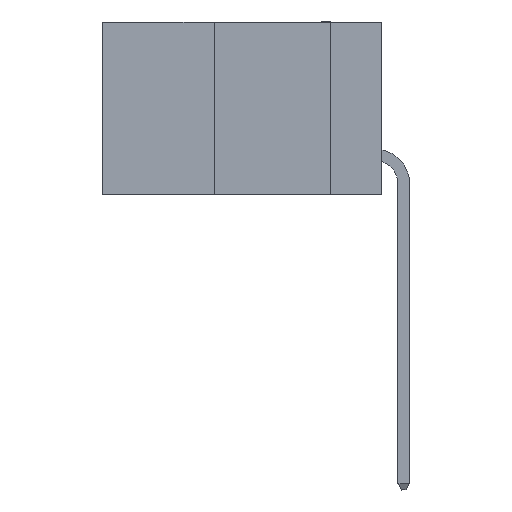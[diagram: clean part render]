
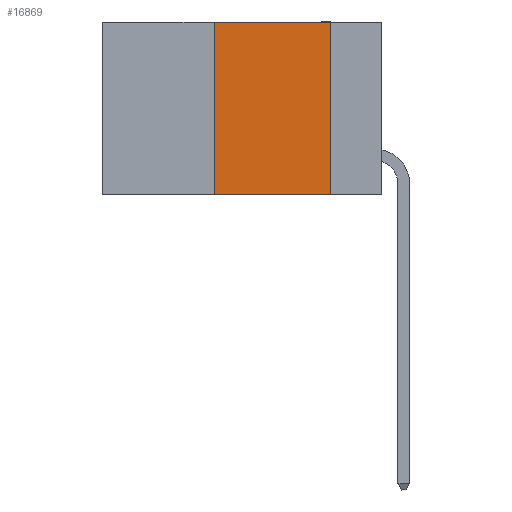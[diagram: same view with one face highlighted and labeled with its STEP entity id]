
A CAD part, left-side view. The second image highlights one B-rep face of the part: STEP entity #16869.
In plain terms, the highlighted planar face has unit normal (-1, 0, 0).
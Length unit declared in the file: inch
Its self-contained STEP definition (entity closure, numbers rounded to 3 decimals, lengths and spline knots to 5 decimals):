
#229 = CARTESIAN_POINT ( 'NONE',  ( 0., 0.36, -0.37 ) ) ;
#3249 = EDGE_CURVE ( 'NONE', #15118, #6403, #12696, .T. ) ;
#6213 = PLANE ( 'NONE',  #23987 ) ;
#6403 = VERTEX_POINT ( 'NONE', #13923 ) ;
#6944 = DIRECTION ( 'NONE',  ( 0., -1., 0. ) ) ;
#7377 = EDGE_LOOP ( 'NONE', ( #34557, #25015, #31800, #25762 ) ) ;
#7876 = CARTESIAN_POINT ( 'NONE',  ( 0., 0.11, 0. ) ) ;
#7880 = VECTOR ( 'NONE', #6944, 39.37008 ) ;
#8492 = EDGE_CURVE ( 'NONE', #6403, #29440, #18945, .T. ) ;
#8942 = DIRECTION ( 'NONE',  ( 0., 0., -1. ) ) ;
#9157 = VECTOR ( 'NONE', #33090, 39.37008 ) ;
#9980 = VERTEX_POINT ( 'NONE', #229 ) ;
#10859 = EDGE_CURVE ( 'NONE', #9980, #15118, #15695, .T. ) ;
#12696 = LINE ( 'NONE', #19470, #9157 ) ;
#13923 = CARTESIAN_POINT ( 'NONE',  ( 0., 0.11, 0. ) ) ;
#15118 = VERTEX_POINT ( 'NONE', #27117 ) ;
#15695 = LINE ( 'NONE', #26704, #30376 ) ;
#16257 = CARTESIAN_POINT ( 'NONE',  ( 0., 0.6, -0.37 ) ) ;
#16719 = VECTOR ( 'NONE', #21004, 39.37008 ) ;
#16869 = ADVANCED_FACE ( 'NONE', ( #17490 ), #6213, .F. ) ;
#17490 = FACE_OUTER_BOUND ( 'NONE', #7377, .T. ) ;
#18259 = DIRECTION ( 'NONE',  ( 0., 0., 1. ) ) ;
#18945 = LINE ( 'NONE', #7876, #16719 ) ;
#19470 = CARTESIAN_POINT ( 'NONE',  ( 0., 0.6, 0. ) ) ;
#21004 = DIRECTION ( 'NONE',  ( 0., 0., -1. ) ) ;
#21558 = EDGE_CURVE ( 'NONE', #9980, #29440, #30498, .T. ) ;
#23987 = AXIS2_PLACEMENT_3D ( 'NONE', #34826, #31999, #8942 ) ;
#25015 = ORIENTED_EDGE ( 'NONE', *, *, #3249, .F. ) ;
#25762 = ORIENTED_EDGE ( 'NONE', *, *, #21558, .T. ) ;
#26704 = CARTESIAN_POINT ( 'NONE',  ( 0., 0.36, 0. ) ) ;
#27117 = CARTESIAN_POINT ( 'NONE',  ( 0., 0.36, 0. ) ) ;
#29440 = VERTEX_POINT ( 'NONE', #31784 ) ;
#30376 = VECTOR ( 'NONE', #18259, 39.37008 ) ;
#30498 = LINE ( 'NONE', #16257, #7880 ) ;
#31784 = CARTESIAN_POINT ( 'NONE',  ( 0., 0.11, -0.37 ) ) ;
#31800 = ORIENTED_EDGE ( 'NONE', *, *, #10859, .F. ) ;
#31999 = DIRECTION ( 'NONE',  ( 1., 0., 0. ) ) ;
#33090 = DIRECTION ( 'NONE',  ( 0., -1., 0. ) ) ;
#34557 = ORIENTED_EDGE ( 'NONE', *, *, #8492, .F. ) ;
#34826 = CARTESIAN_POINT ( 'NONE',  ( 0., 0.6, 0. ) ) ;
